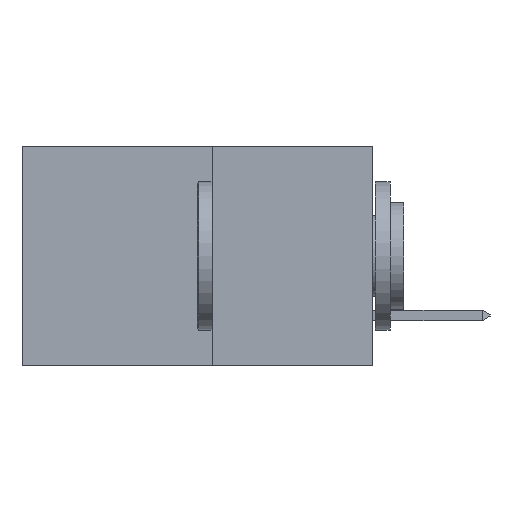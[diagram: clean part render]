
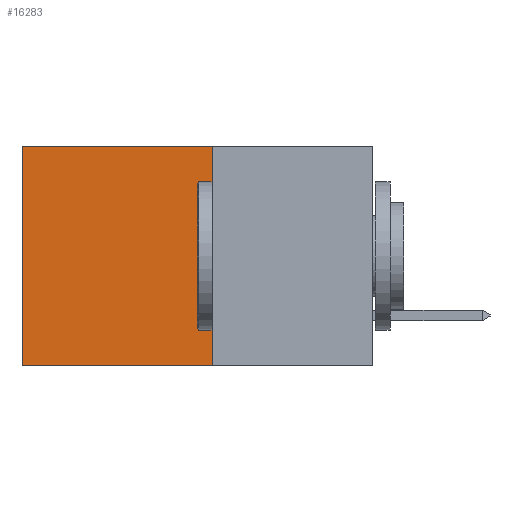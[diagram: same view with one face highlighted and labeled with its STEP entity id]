
A CAD part, left-side view. The second image highlights one B-rep face of the part: STEP entity #16283.
In plain terms, the highlighted planar face has unit normal (-1, 0, 0).
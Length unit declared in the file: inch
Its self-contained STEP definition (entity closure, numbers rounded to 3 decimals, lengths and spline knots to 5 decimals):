
#48 = DIRECTION ( 'NONE',  ( 0., 1., 0. ) ) ;
#1704 = EDGE_CURVE ( 'NONE', #7356, #14299, #3898, .T. ) ;
#2830 = LINE ( 'NONE', #19964, #17126 ) ;
#3110 = VERTEX_POINT ( 'NONE', #3720 ) ;
#3720 = CARTESIAN_POINT ( 'NONE',  ( 0.277, 0.59, 0. ) ) ;
#3825 = CARTESIAN_POINT ( 'NONE',  ( 0.277, 0.27, 0. ) ) ;
#3898 = LINE ( 'NONE', #18893, #13868 ) ;
#3923 = DIRECTION ( 'NONE',  ( 1., 0., 0. ) ) ;
#4689 = LINE ( 'NONE', #4926, #10354 ) ;
#4926 = CARTESIAN_POINT ( 'NONE',  ( 0.277, 0.59, -0.37 ) ) ;
#5143 = DIRECTION ( 'NONE',  ( 0., 1., 0. ) ) ;
#6244 = CARTESIAN_POINT ( 'NONE',  ( 0.277, 0.59, -0.37 ) ) ;
#6721 = EDGE_CURVE ( 'NONE', #3110, #14299, #4689, .T. ) ;
#7356 = VERTEX_POINT ( 'NONE', #23399 ) ;
#7803 = AXIS2_PLACEMENT_3D ( 'NONE', #15127, #3923, #16963 ) ;
#8712 = DIRECTION ( 'NONE',  ( 0., 0., -1. ) ) ;
#9336 = CARTESIAN_POINT ( 'NONE',  ( 0.277, 0.27, -0.37 ) ) ;
#9712 = EDGE_CURVE ( 'NONE', #13460, #3110, #2830, .T. ) ;
#10354 = VECTOR ( 'NONE', #8712, 39.37008 ) ;
#10556 = EDGE_CURVE ( 'NONE', #13460, #7356, #17075, .T. ) ;
#12870 = ORIENTED_EDGE ( 'NONE', *, *, #10556, .F. ) ;
#13246 = PLANE ( 'NONE',  #7803 ) ;
#13460 = VERTEX_POINT ( 'NONE', #3825 ) ;
#13868 = VECTOR ( 'NONE', #48, 39.37008 ) ;
#14299 = VERTEX_POINT ( 'NONE', #6244 ) ;
#15127 = CARTESIAN_POINT ( 'NONE',  ( 0.277, 0.27, -0.37 ) ) ;
#16071 = EDGE_LOOP ( 'NONE', ( #21356, #16120, #12870, #21444 ) ) ;
#16120 = ORIENTED_EDGE ( 'NONE', *, *, #1704, .F. ) ;
#16283 = ADVANCED_FACE ( 'NONE', ( #22858 ), #13246, .F. ) ;
#16963 = DIRECTION ( 'NONE',  ( 0., 0., -1. ) ) ;
#17075 = LINE ( 'NONE', #9336, #21862 ) ;
#17126 = VECTOR ( 'NONE', #5143, 39.37008 ) ;
#18893 = CARTESIAN_POINT ( 'NONE',  ( 0.277, 0.27, -0.37 ) ) ;
#19964 = CARTESIAN_POINT ( 'NONE',  ( 0.277, 0.27, 0. ) ) ;
#21356 = ORIENTED_EDGE ( 'NONE', *, *, #6721, .T. ) ;
#21444 = ORIENTED_EDGE ( 'NONE', *, *, #9712, .T. ) ;
#21862 = VECTOR ( 'NONE', #22206, 39.37008 ) ;
#22206 = DIRECTION ( 'NONE',  ( 0., 0., -1. ) ) ;
#22858 = FACE_OUTER_BOUND ( 'NONE', #16071, .T. ) ;
#23399 = CARTESIAN_POINT ( 'NONE',  ( 0.277, 0.27, -0.37 ) ) ;
